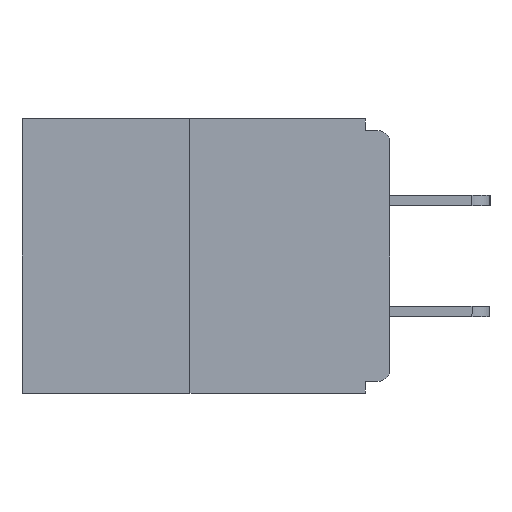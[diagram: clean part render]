
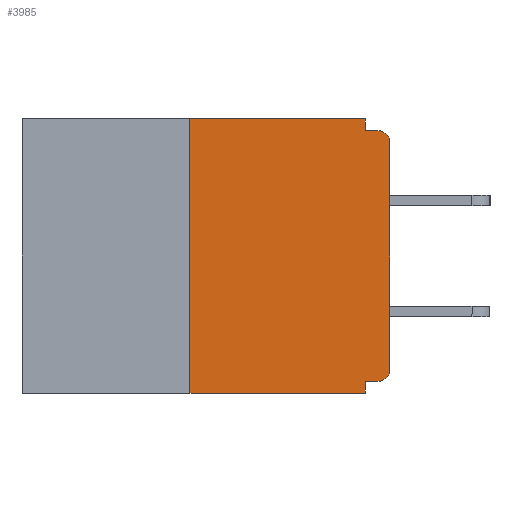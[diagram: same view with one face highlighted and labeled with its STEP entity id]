
A CAD part, left-side view. The second image highlights one B-rep face of the part: STEP entity #3985.
In plain terms, the highlighted planar face has unit normal (-1, 0, 0).
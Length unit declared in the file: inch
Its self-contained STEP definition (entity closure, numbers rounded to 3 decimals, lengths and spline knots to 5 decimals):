
#575 = DIRECTION ( 'NONE',  ( 0., 0., -1. ) ) ;
#684 = CARTESIAN_POINT ( 'NONE',  ( 0., 0.031, 0. ) ) ;
#711 = CIRCLE ( 'NONE', #7188, 0.015 ) ;
#1336 = VERTEX_POINT ( 'NONE', #5161 ) ;
#1677 = EDGE_CURVE ( 'NONE', #9394, #4862, #17763, .T. ) ;
#2064 = ORIENTED_EDGE ( 'NONE', *, *, #9178, .T. ) ;
#2186 = ORIENTED_EDGE ( 'NONE', *, *, #9922, .F. ) ;
#2549 = CARTESIAN_POINT ( 'NONE',  ( 0., 0.25, -0.343 ) ) ;
#2891 = DIRECTION ( 'NONE',  ( 1., 0., 0. ) ) ;
#3330 = DIRECTION ( 'NONE',  ( 0., 0., -1. ) ) ;
#3423 = CARTESIAN_POINT ( 'NONE',  ( 0., 0.015, -0.313 ) ) ;
#3985 = ADVANCED_FACE ( 'NONE', ( #8352 ), #23733, .F. ) ;
#4031 = CARTESIAN_POINT ( 'NONE',  ( 0., 0.031, -0.343 ) ) ;
#4551 = EDGE_CURVE ( 'NONE', #25738, #9394, #14948, .T. ) ;
#4862 = VERTEX_POINT ( 'NONE', #19441 ) ;
#5161 = CARTESIAN_POINT ( 'NONE',  ( 0., 0.031, -0.015 ) ) ;
#5474 = LINE ( 'NONE', #19102, #23290 ) ;
#6037 = EDGE_CURVE ( 'NONE', #26537, #13484, #5474, .T. ) ;
#6187 = ORIENTED_EDGE ( 'NONE', *, *, #26991, .T. ) ;
#6196 = VECTOR ( 'NONE', #9642, 39.37008 ) ;
#6480 = DIRECTION ( 'NONE',  ( 0., 0., 1. ) ) ;
#6794 = DIRECTION ( 'NONE',  ( 0., -1., 0. ) ) ;
#6859 = LINE ( 'NONE', #23854, #14750 ) ;
#7188 = AXIS2_PLACEMENT_3D ( 'NONE', #3423, #9439, #3330 ) ;
#7221 = ORIENTED_EDGE ( 'NONE', *, *, #11243, .F. ) ;
#7553 = ORIENTED_EDGE ( 'NONE', *, *, #8041, .T. ) ;
#7763 = CARTESIAN_POINT ( 'NONE',  ( 0., 0.46, -0.343 ) ) ;
#8041 = EDGE_CURVE ( 'NONE', #10546, #19221, #13909, .T. ) ;
#8352 = FACE_OUTER_BOUND ( 'NONE', #18716, .T. ) ;
#8725 = VERTEX_POINT ( 'NONE', #23002 ) ;
#8844 = DIRECTION ( 'NONE',  ( 0., 0., -1. ) ) ;
#9027 = CARTESIAN_POINT ( 'NONE',  ( 0., 0.031, 0. ) ) ;
#9178 = EDGE_CURVE ( 'NONE', #25738, #10546, #711, .T. ) ;
#9394 = VERTEX_POINT ( 'NONE', #12633 ) ;
#9439 = DIRECTION ( 'NONE',  ( -1., 0., 0. ) ) ;
#9641 = VECTOR ( 'NONE', #15531, 39.37008 ) ;
#9642 = DIRECTION ( 'NONE',  ( 0., -1., 0. ) ) ;
#9922 = EDGE_CURVE ( 'NONE', #13484, #19414, #14842, .T. ) ;
#10445 = AXIS2_PLACEMENT_3D ( 'NONE', #14778, #22814, #21068 ) ;
#10546 = VERTEX_POINT ( 'NONE', #23249 ) ;
#10658 = CIRCLE ( 'NONE', #10445, 0.015 ) ;
#11243 = EDGE_CURVE ( 'NONE', #1336, #8725, #6859, .T. ) ;
#11744 = VECTOR ( 'NONE', #8844, 39.37008 ) ;
#12633 = CARTESIAN_POINT ( 'NONE',  ( 0., 0.031, -0.328 ) ) ;
#13484 = VERTEX_POINT ( 'NONE', #17589 ) ;
#13778 = DIRECTION ( 'NONE',  ( 0., -1., 0. ) ) ;
#13909 = LINE ( 'NONE', #24195, #9641 ) ;
#14008 = ORIENTED_EDGE ( 'NONE', *, *, #24783, .F. ) ;
#14750 = VECTOR ( 'NONE', #13778, 39.37008 ) ;
#14778 = CARTESIAN_POINT ( 'NONE',  ( 0., 0.015, -0.03 ) ) ;
#14842 = LINE ( 'NONE', #21734, #24395 ) ;
#14948 = LINE ( 'NONE', #18147, #21907 ) ;
#15283 = ORIENTED_EDGE ( 'NONE', *, *, #1677, .F. ) ;
#15531 = DIRECTION ( 'NONE',  ( 0., 0., 1. ) ) ;
#15564 = AXIS2_PLACEMENT_3D ( 'NONE', #23994, #2891, #575 ) ;
#17589 = CARTESIAN_POINT ( 'NONE',  ( 0., 0.25, 0. ) ) ;
#17763 = LINE ( 'NONE', #4031, #23693 ) ;
#18147 = CARTESIAN_POINT ( 'NONE',  ( 0., 0., -0.328 ) ) ;
#18255 = ORIENTED_EDGE ( 'NONE', *, *, #4551, .F. ) ;
#18618 = CARTESIAN_POINT ( 'NONE',  ( 0., 0.015, -0.328 ) ) ;
#18716 = EDGE_LOOP ( 'NONE', ( #2186, #21717, #21367, #15283, #18255, #2064, #7553, #6187, #7221, #14008 ) ) ;
#19102 = CARTESIAN_POINT ( 'NONE',  ( 0., 0.25, 0. ) ) ;
#19221 = VERTEX_POINT ( 'NONE', #25528 ) ;
#19414 = VERTEX_POINT ( 'NONE', #684 ) ;
#19441 = CARTESIAN_POINT ( 'NONE',  ( 0., 0.031, -0.343 ) ) ;
#19738 = EDGE_CURVE ( 'NONE', #26537, #4862, #23035, .T. ) ;
#21068 = DIRECTION ( 'NONE',  ( 0., 0., -1. ) ) ;
#21367 = ORIENTED_EDGE ( 'NONE', *, *, #19738, .T. ) ;
#21717 = ORIENTED_EDGE ( 'NONE', *, *, #6037, .F. ) ;
#21734 = CARTESIAN_POINT ( 'NONE',  ( 0., 0.46, 0. ) ) ;
#21907 = VECTOR ( 'NONE', #24231, 39.37008 ) ;
#22814 = DIRECTION ( 'NONE',  ( -1., 0., 0. ) ) ;
#23002 = CARTESIAN_POINT ( 'NONE',  ( 0., 0.015, -0.015 ) ) ;
#23035 = LINE ( 'NONE', #7763, #6196 ) ;
#23249 = CARTESIAN_POINT ( 'NONE',  ( 0., 0., -0.313 ) ) ;
#23290 = VECTOR ( 'NONE', #6480, 39.37008 ) ;
#23693 = VECTOR ( 'NONE', #25346, 39.37008 ) ;
#23733 = PLANE ( 'NONE',  #15564 ) ;
#23854 = CARTESIAN_POINT ( 'NONE',  ( 0., 0., -0.015 ) ) ;
#23994 = CARTESIAN_POINT ( 'NONE',  ( 0., 0.46, 0. ) ) ;
#24195 = CARTESIAN_POINT ( 'NONE',  ( 0., 0., 0. ) ) ;
#24231 = DIRECTION ( 'NONE',  ( 0., 1., 0. ) ) ;
#24395 = VECTOR ( 'NONE', #6794, 39.37008 ) ;
#24783 = EDGE_CURVE ( 'NONE', #19414, #1336, #26951, .T. ) ;
#25346 = DIRECTION ( 'NONE',  ( 0., 0., -1. ) ) ;
#25528 = CARTESIAN_POINT ( 'NONE',  ( 0., 0., -0.03 ) ) ;
#25738 = VERTEX_POINT ( 'NONE', #18618 ) ;
#26537 = VERTEX_POINT ( 'NONE', #2549 ) ;
#26951 = LINE ( 'NONE', #9027, #11744 ) ;
#26991 = EDGE_CURVE ( 'NONE', #19221, #8725, #10658, .T. ) ;
